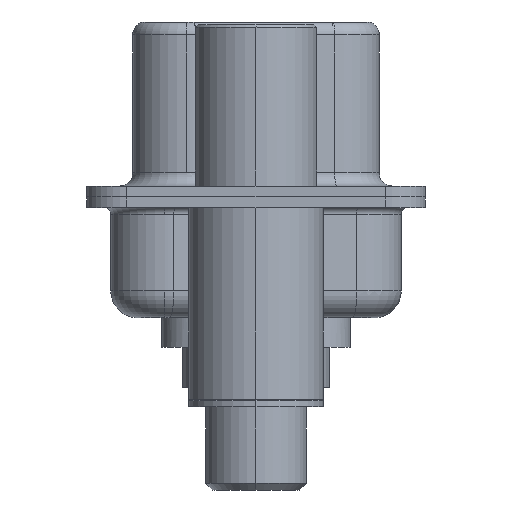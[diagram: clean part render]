
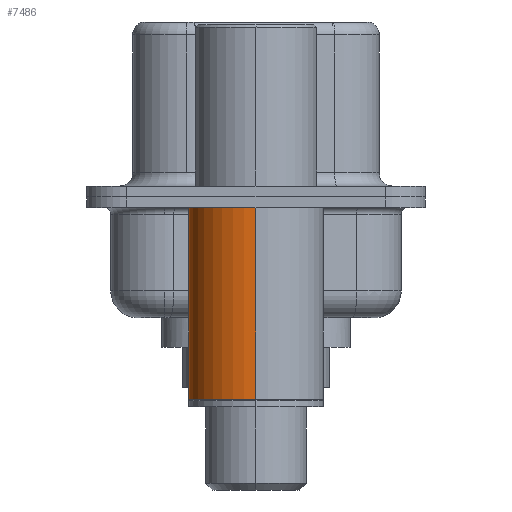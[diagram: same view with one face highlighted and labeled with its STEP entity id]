
A CAD part, left-side view. The second image highlights one B-rep face of the part: STEP entity #7486.
In plain terms, the highlighted cylindrical face has radius 2.5 mm (diameter 5 mm), a partial arc.
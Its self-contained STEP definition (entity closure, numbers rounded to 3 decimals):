
#79 = EDGE_CURVE ( 'NONE', #11972, #2916, #14889, .T. ) ;
#281 = CARTESIAN_POINT ( 'NONE',  ( 2.5, 0., -7.525 ) ) ;
#358 = CIRCLE ( 'NONE', #5291, 2.5 ) ;
#606 = ORIENTED_EDGE ( 'NONE', *, *, #15930, .T. ) ;
#1066 = EDGE_LOOP ( 'NONE', ( #606, #16314, #1099, #12426 ) ) ;
#1099 = ORIENTED_EDGE ( 'NONE', *, *, #14515, .F. ) ;
#1300 = CARTESIAN_POINT ( 'NONE',  ( -2.5, 0., -0.4 ) ) ;
#1408 = CARTESIAN_POINT ( 'NONE',  ( 0., 0., -7.525 ) ) ;
#1595 = CIRCLE ( 'NONE', #15968, 2.5 ) ;
#2792 = DIRECTION ( 'NONE',  ( 0., 0., 1. ) ) ;
#2826 = CARTESIAN_POINT ( 'NONE',  ( 2.5, 0., 0.581 ) ) ;
#2829 = VERTEX_POINT ( 'NONE', #1300 ) ;
#2916 = VERTEX_POINT ( 'NONE', #4610 ) ;
#3925 = EDGE_CURVE ( 'NONE', #13026, #2829, #6871, .T. ) ;
#3972 = CARTESIAN_POINT ( 'NONE',  ( 0., 0., 0.581 ) ) ;
#4610 = CARTESIAN_POINT ( 'NONE',  ( 2.5, 0., -0.4 ) ) ;
#5291 = AXIS2_PLACEMENT_3D ( 'NONE', #12476, #12644, #16687 ) ;
#6871 = LINE ( 'NONE', #15555, #12684 ) ;
#7486 = ADVANCED_FACE ( 'NONE', ( #17828 ), #15663, .T. ) ;
#9328 = CARTESIAN_POINT ( 'NONE',  ( -2.5, 0., -7.525 ) ) ;
#9941 = DIRECTION ( 'NONE',  ( 0., 0., 1. ) ) ;
#11972 = VERTEX_POINT ( 'NONE', #281 ) ;
#12426 = ORIENTED_EDGE ( 'NONE', *, *, #79, .F. ) ;
#12476 = CARTESIAN_POINT ( 'NONE',  ( 0., 0., -0.4 ) ) ;
#12515 = DIRECTION ( 'NONE',  ( 1., 0., 0. ) ) ;
#12644 = DIRECTION ( 'NONE',  ( 0., 0., 1. ) ) ;
#12684 = VECTOR ( 'NONE', #9941, 1000. ) ;
#13026 = VERTEX_POINT ( 'NONE', #9328 ) ;
#13678 = DIRECTION ( 'NONE',  ( 1., 0., 0. ) ) ;
#14515 = EDGE_CURVE ( 'NONE', #2916, #2829, #358, .T. ) ;
#14870 = VECTOR ( 'NONE', #16464, 1000. ) ;
#14889 = LINE ( 'NONE', #2826, #14870 ) ;
#15555 = CARTESIAN_POINT ( 'NONE',  ( -2.5, 0., 0.581 ) ) ;
#15663 = CYLINDRICAL_SURFACE ( 'NONE', #17977, 2.5 ) ;
#15930 = EDGE_CURVE ( 'NONE', #11972, #13026, #1595, .T. ) ;
#15968 = AXIS2_PLACEMENT_3D ( 'NONE', #1408, #2792, #12515 ) ;
#16314 = ORIENTED_EDGE ( 'NONE', *, *, #3925, .T. ) ;
#16464 = DIRECTION ( 'NONE',  ( 0., 0., 1. ) ) ;
#16687 = DIRECTION ( 'NONE',  ( 1., 0., 0. ) ) ;
#17828 = FACE_OUTER_BOUND ( 'NONE', #1066, .T. ) ;
#17939 = DIRECTION ( 'NONE',  ( 0., 0., 1. ) ) ;
#17977 = AXIS2_PLACEMENT_3D ( 'NONE', #3972, #17939, #13678 ) ;
